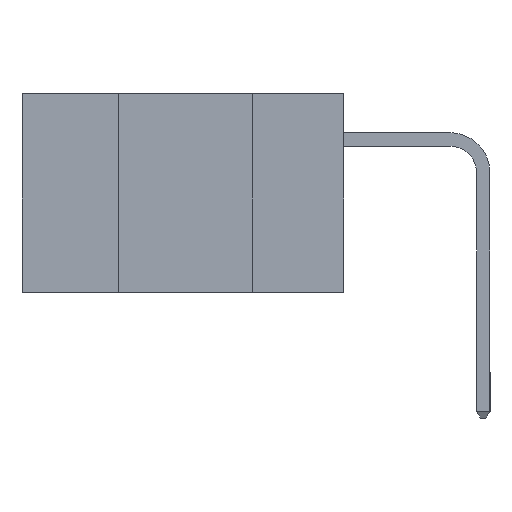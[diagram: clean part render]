
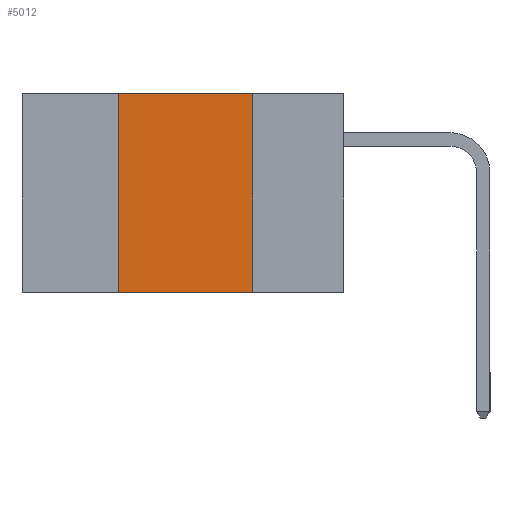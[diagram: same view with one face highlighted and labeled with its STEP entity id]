
A CAD part, left-side view. The second image highlights one B-rep face of the part: STEP entity #5012.
In plain terms, the highlighted planar face has unit normal (-1, 0, 0).
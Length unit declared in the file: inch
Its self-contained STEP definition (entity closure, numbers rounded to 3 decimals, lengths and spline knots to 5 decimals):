
#110 = DIRECTION ( 'NONE',  ( 0., -1., 0. ) ) ;
#671 = LINE ( 'NONE', #1959, #6470 ) ;
#688 = VERTEX_POINT ( 'NONE', #7592 ) ;
#922 = LINE ( 'NONE', #5271, #9273 ) ;
#1242 = DIRECTION ( 'NONE',  ( 0., 0., 1. ) ) ;
#1400 = DIRECTION ( 'NONE',  ( 0., -1., 0. ) ) ;
#1778 = CARTESIAN_POINT ( 'NONE',  ( 0., 0.17, -0.37 ) ) ;
#1959 = CARTESIAN_POINT ( 'NONE',  ( 0., 0.17, 0. ) ) ;
#1962 = ORIENTED_EDGE ( 'NONE', *, *, #2390, .F. ) ;
#2127 = CARTESIAN_POINT ( 'NONE',  ( 0., 0.6, 0. ) ) ;
#2390 = EDGE_CURVE ( 'NONE', #6245, #5982, #2973, .T. ) ;
#2973 = LINE ( 'NONE', #2127, #9845 ) ;
#3276 = ORIENTED_EDGE ( 'NONE', *, *, #3651, .T. ) ;
#3651 = EDGE_CURVE ( 'NONE', #688, #7987, #922, .T. ) ;
#3733 = EDGE_LOOP ( 'NONE', ( #6578, #1962, #8569, #3276 ) ) ;
#3866 = DIRECTION ( 'NONE',  ( 0., 0., -1. ) ) ;
#4410 = CARTESIAN_POINT ( 'NONE',  ( 0., 0.6, 0. ) ) ;
#4811 = CARTESIAN_POINT ( 'NONE',  ( 0., 0.17, 0. ) ) ;
#5012 = ADVANCED_FACE ( 'NONE', ( #8860 ), #8713, .F. ) ;
#5102 = CARTESIAN_POINT ( 'NONE',  ( 0., 0.42, 0. ) ) ;
#5271 = CARTESIAN_POINT ( 'NONE',  ( 0., 0.6, -0.37 ) ) ;
#5402 = DIRECTION ( 'NONE',  ( 0., 0., -1. ) ) ;
#5546 = CARTESIAN_POINT ( 'NONE',  ( 0., 0.42, 0. ) ) ;
#5805 = VECTOR ( 'NONE', #1242, 39.37008 ) ;
#5932 = LINE ( 'NONE', #5546, #5805 ) ;
#5982 = VERTEX_POINT ( 'NONE', #4811 ) ;
#6245 = VERTEX_POINT ( 'NONE', #5102 ) ;
#6470 = VECTOR ( 'NONE', #3866, 39.37008 ) ;
#6578 = ORIENTED_EDGE ( 'NONE', *, *, #8888, .F. ) ;
#7592 = CARTESIAN_POINT ( 'NONE',  ( 0., 0.42, -0.37 ) ) ;
#7905 = AXIS2_PLACEMENT_3D ( 'NONE', #4410, #8864, #5402 ) ;
#7987 = VERTEX_POINT ( 'NONE', #1778 ) ;
#8569 = ORIENTED_EDGE ( 'NONE', *, *, #8858, .F. ) ;
#8713 = PLANE ( 'NONE',  #7905 ) ;
#8858 = EDGE_CURVE ( 'NONE', #688, #6245, #5932, .T. ) ;
#8860 = FACE_OUTER_BOUND ( 'NONE', #3733, .T. ) ;
#8864 = DIRECTION ( 'NONE',  ( 1., 0., 0. ) ) ;
#8888 = EDGE_CURVE ( 'NONE', #5982, #7987, #671, .T. ) ;
#9273 = VECTOR ( 'NONE', #110, 39.37008 ) ;
#9845 = VECTOR ( 'NONE', #1400, 39.37008 ) ;
